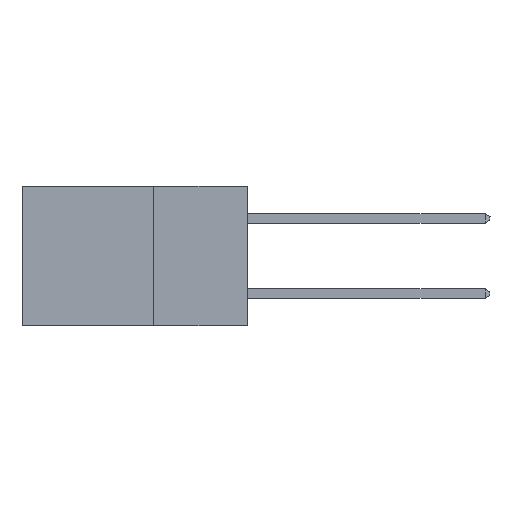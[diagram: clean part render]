
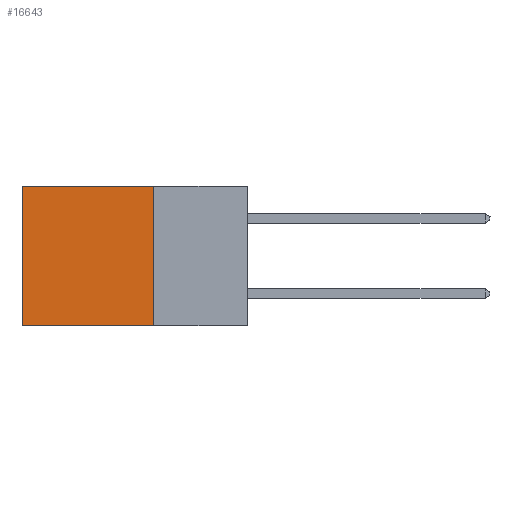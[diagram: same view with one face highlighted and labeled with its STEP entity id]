
A CAD part, left-side view. The second image highlights one B-rep face of the part: STEP entity #16643.
In plain terms, the highlighted planar face has unit normal (-1, 0, 0).
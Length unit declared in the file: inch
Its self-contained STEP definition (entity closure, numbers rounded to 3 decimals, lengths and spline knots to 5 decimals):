
#684 = LINE ( 'NONE', #7237, #10003 ) ;
#1285 = ORIENTED_EDGE ( 'NONE', *, *, #6401, .F. ) ;
#2713 = DIRECTION ( 'NONE',  ( 0., 0., -1. ) ) ;
#2792 = VERTEX_POINT ( 'NONE', #20851 ) ;
#4331 = FACE_OUTER_BOUND ( 'NONE', #12392, .T. ) ;
#4468 = LINE ( 'NONE', #5922, #13830 ) ;
#4620 = CARTESIAN_POINT ( 'NONE',  ( 0.298, 0.25, -0.37 ) ) ;
#5362 = LINE ( 'NONE', #13654, #18531 ) ;
#5674 = DIRECTION ( 'NONE',  ( 0., 0., -1. ) ) ;
#5922 = CARTESIAN_POINT ( 'NONE',  ( 0.298, 0.25, 0. ) ) ;
#6005 = PLANE ( 'NONE',  #12690 ) ;
#6401 = EDGE_CURVE ( 'NONE', #24158, #17592, #684, .T. ) ;
#6881 = CARTESIAN_POINT ( 'NONE',  ( 0.298, 0.25, 0. ) ) ;
#7237 = CARTESIAN_POINT ( 'NONE',  ( 0.298, 0.25, -0.37 ) ) ;
#7534 = CARTESIAN_POINT ( 'NONE',  ( 0.298, 0.6, 0. ) ) ;
#7835 = VERTEX_POINT ( 'NONE', #6881 ) ;
#8084 = DIRECTION ( 'NONE',  ( 0., 1., 0. ) ) ;
#9059 = ORIENTED_EDGE ( 'NONE', *, *, #14199, .F. ) ;
#9436 = ORIENTED_EDGE ( 'NONE', *, *, #22086, .T. ) ;
#9669 = CARTESIAN_POINT ( 'NONE',  ( 0.298, 0.25, 0. ) ) ;
#10003 = VECTOR ( 'NONE', #18145, 39.37008 ) ;
#11229 = ORIENTED_EDGE ( 'NONE', *, *, #13839, .T. ) ;
#11361 = CARTESIAN_POINT ( 'NONE',  ( 0.298, 0.6, -0.37 ) ) ;
#12392 = EDGE_LOOP ( 'NONE', ( #9436, #1285, #9059, #11229 ) ) ;
#12690 = AXIS2_PLACEMENT_3D ( 'NONE', #9669, #21000, #20915 ) ;
#13654 = CARTESIAN_POINT ( 'NONE',  ( 0.298, 0.25, 0. ) ) ;
#13830 = VECTOR ( 'NONE', #5674, 39.37008 ) ;
#13839 = EDGE_CURVE ( 'NONE', #7835, #2792, #5362, .T. ) ;
#14199 = EDGE_CURVE ( 'NONE', #7835, #24158, #4468, .T. ) ;
#16643 = ADVANCED_FACE ( 'NONE', ( #4331 ), #6005, .F. ) ;
#17588 = VECTOR ( 'NONE', #2713, 39.37008 ) ;
#17592 = VERTEX_POINT ( 'NONE', #11361 ) ;
#18145 = DIRECTION ( 'NONE',  ( 0., 1., 0. ) ) ;
#18531 = VECTOR ( 'NONE', #8084, 39.37008 ) ;
#19632 = LINE ( 'NONE', #7534, #17588 ) ;
#20851 = CARTESIAN_POINT ( 'NONE',  ( 0.298, 0.6, 0. ) ) ;
#20915 = DIRECTION ( 'NONE',  ( 0., 0., -1. ) ) ;
#21000 = DIRECTION ( 'NONE',  ( 1., 0., 0. ) ) ;
#22086 = EDGE_CURVE ( 'NONE', #2792, #17592, #19632, .T. ) ;
#24158 = VERTEX_POINT ( 'NONE', #4620 ) ;
